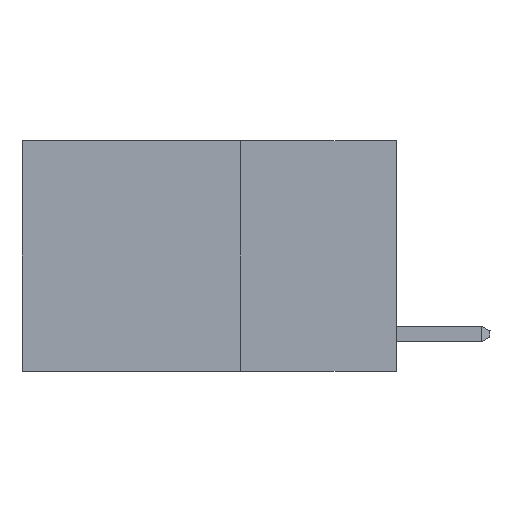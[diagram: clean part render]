
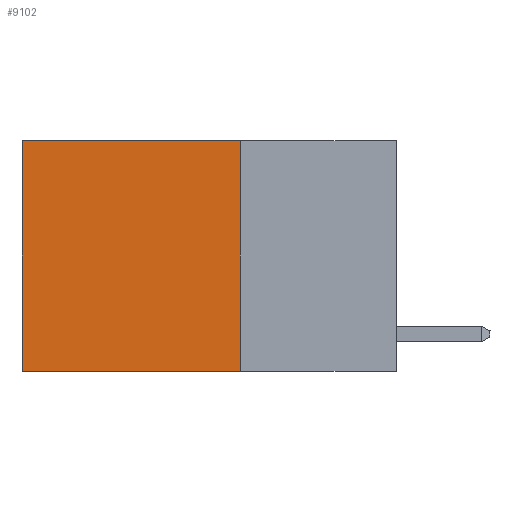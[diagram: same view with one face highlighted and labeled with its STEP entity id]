
A CAD part, left-side view. The second image highlights one B-rep face of the part: STEP entity #9102.
In plain terms, the highlighted planar face has unit normal (-1, 0, 0).
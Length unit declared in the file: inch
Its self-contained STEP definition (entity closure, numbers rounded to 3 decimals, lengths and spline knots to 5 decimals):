
#92 = DIRECTION ( 'NONE',  ( 1., 0., 0. ) ) ;
#200 = VECTOR ( 'NONE', #7847, 39.37008 ) ;
#445 = CARTESIAN_POINT ( 'NONE',  ( 0.2625, 0.25, 0. ) ) ;
#668 = ORIENTED_EDGE ( 'NONE', *, *, #8061, .F. ) ;
#925 = CARTESIAN_POINT ( 'NONE',  ( 0.2625, 0.6, 0. ) ) ;
#1306 = DIRECTION ( 'NONE',  ( 0., 0., -1. ) ) ;
#1818 = EDGE_CURVE ( 'NONE', #5085, #8027, #13480, .T. ) ;
#1957 = VECTOR ( 'NONE', #7352, 39.37008 ) ;
#2193 = CARTESIAN_POINT ( 'NONE',  ( 0.2625, 0.25, -0.37 ) ) ;
#2200 = ORIENTED_EDGE ( 'NONE', *, *, #1818, .T. ) ;
#2342 = CARTESIAN_POINT ( 'NONE',  ( 0.2625, 0.25, 0. ) ) ;
#2468 = CARTESIAN_POINT ( 'NONE',  ( 0.2625, 0.6, -0.37 ) ) ;
#5085 = VERTEX_POINT ( 'NONE', #445 ) ;
#5869 = VECTOR ( 'NONE', #11823, 39.37008 ) ;
#6635 = VERTEX_POINT ( 'NONE', #2468 ) ;
#6685 = VECTOR ( 'NONE', #1306, 39.37008 ) ;
#7109 = AXIS2_PLACEMENT_3D ( 'NONE', #13284, #92, #14467 ) ;
#7131 = CARTESIAN_POINT ( 'NONE',  ( 0.2625, 0.6, 0. ) ) ;
#7352 = DIRECTION ( 'NONE',  ( 0., 1., 0. ) ) ;
#7847 = DIRECTION ( 'NONE',  ( 0., 0., -1. ) ) ;
#8027 = VERTEX_POINT ( 'NONE', #925 ) ;
#8061 = EDGE_CURVE ( 'NONE', #11842, #6635, #13789, .T. ) ;
#8795 = ORIENTED_EDGE ( 'NONE', *, *, #9447, .F. ) ;
#8858 = LINE ( 'NONE', #13746, #200 ) ;
#9102 = ADVANCED_FACE ( 'NONE', ( #14344 ), #12099, .F. ) ;
#9145 = CARTESIAN_POINT ( 'NONE',  ( 0.2625, 0.25, -0.37 ) ) ;
#9447 = EDGE_CURVE ( 'NONE', #5085, #11842, #8858, .T. ) ;
#9914 = LINE ( 'NONE', #7131, #6685 ) ;
#11823 = DIRECTION ( 'NONE',  ( 0., 1., 0. ) ) ;
#11842 = VERTEX_POINT ( 'NONE', #9145 ) ;
#12099 = PLANE ( 'NONE',  #7109 ) ;
#12839 = EDGE_CURVE ( 'NONE', #8027, #6635, #9914, .T. ) ;
#13284 = CARTESIAN_POINT ( 'NONE',  ( 0.2625, 0.25, 0. ) ) ;
#13480 = LINE ( 'NONE', #2342, #1957 ) ;
#13746 = CARTESIAN_POINT ( 'NONE',  ( 0.2625, 0.25, 0. ) ) ;
#13789 = LINE ( 'NONE', #2193, #5869 ) ;
#14203 = EDGE_LOOP ( 'NONE', ( #14701, #668, #8795, #2200 ) ) ;
#14344 = FACE_OUTER_BOUND ( 'NONE', #14203, .T. ) ;
#14467 = DIRECTION ( 'NONE',  ( 0., 0., -1. ) ) ;
#14701 = ORIENTED_EDGE ( 'NONE', *, *, #12839, .T. ) ;
